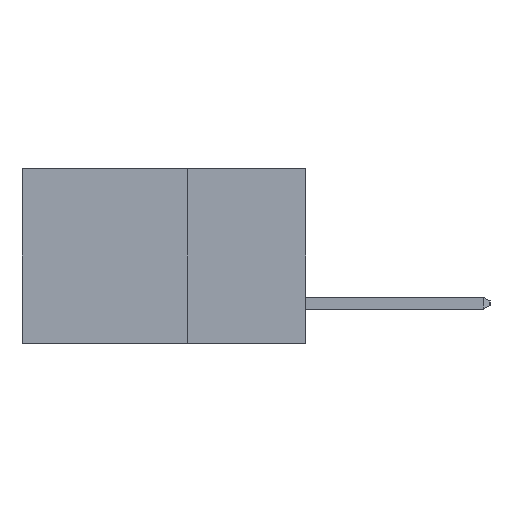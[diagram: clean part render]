
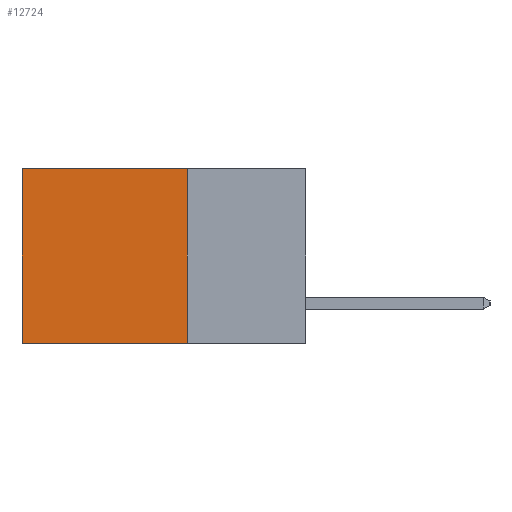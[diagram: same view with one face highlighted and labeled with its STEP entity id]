
A CAD part, left-side view. The second image highlights one B-rep face of the part: STEP entity #12724.
In plain terms, the highlighted planar face has unit normal (-1, 0, 0).
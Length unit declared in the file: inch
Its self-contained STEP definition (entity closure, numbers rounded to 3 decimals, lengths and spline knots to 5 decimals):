
#132 = CARTESIAN_POINT ( 'NONE',  ( 0.298, 0.25, 0. ) ) ;
#136 = ORIENTED_EDGE ( 'NONE', *, *, #9781, .F. ) ;
#365 = ORIENTED_EDGE ( 'NONE', *, *, #11097, .F. ) ;
#1164 = VERTEX_POINT ( 'NONE', #7019 ) ;
#1993 = EDGE_CURVE ( 'NONE', #12149, #13984, #2616, .T. ) ;
#2065 = AXIS2_PLACEMENT_3D ( 'NONE', #5774, #7041, #15264 ) ;
#2164 = EDGE_CURVE ( 'NONE', #5030, #12149, #10288, .T. ) ;
#2616 = LINE ( 'NONE', #6552, #8946 ) ;
#2800 = VECTOR ( 'NONE', #10578, 39.37008 ) ;
#4017 = CARTESIAN_POINT ( 'NONE',  ( 0.298, 0.25, 0. ) ) ;
#4570 = CARTESIAN_POINT ( 'NONE',  ( 0.298, 0.6, 0. ) ) ;
#5030 = VERTEX_POINT ( 'NONE', #132 ) ;
#5410 = LINE ( 'NONE', #13071, #11493 ) ;
#5774 = CARTESIAN_POINT ( 'NONE',  ( 0.298, 0.25, 0. ) ) ;
#6486 = DIRECTION ( 'NONE',  ( 0., 0., -1. ) ) ;
#6552 = CARTESIAN_POINT ( 'NONE',  ( 0.298, 0.6, 0. ) ) ;
#7019 = CARTESIAN_POINT ( 'NONE',  ( 0.298, 0.25, -0.37 ) ) ;
#7041 = DIRECTION ( 'NONE',  ( 1., 0., 0. ) ) ;
#7250 = DIRECTION ( 'NONE',  ( 0., 1., 0. ) ) ;
#7661 = EDGE_LOOP ( 'NONE', ( #11614, #365, #136, #7748 ) ) ;
#7748 = ORIENTED_EDGE ( 'NONE', *, *, #2164, .T. ) ;
#8946 = VECTOR ( 'NONE', #6486, 39.37008 ) ;
#9781 = EDGE_CURVE ( 'NONE', #5030, #1164, #15673, .T. ) ;
#10288 = LINE ( 'NONE', #4017, #12952 ) ;
#10578 = DIRECTION ( 'NONE',  ( 0., 0., -1. ) ) ;
#10664 = CARTESIAN_POINT ( 'NONE',  ( 0.298, 0.25, 0. ) ) ;
#11097 = EDGE_CURVE ( 'NONE', #1164, #13984, #5410, .T. ) ;
#11460 = FACE_OUTER_BOUND ( 'NONE', #7661, .T. ) ;
#11493 = VECTOR ( 'NONE', #12766, 39.37008 ) ;
#11614 = ORIENTED_EDGE ( 'NONE', *, *, #1993, .T. ) ;
#11801 = CARTESIAN_POINT ( 'NONE',  ( 0.298, 0.6, -0.37 ) ) ;
#12149 = VERTEX_POINT ( 'NONE', #4570 ) ;
#12724 = ADVANCED_FACE ( 'NONE', ( #11460 ), #12906, .F. ) ;
#12766 = DIRECTION ( 'NONE',  ( 0., 1., 0. ) ) ;
#12906 = PLANE ( 'NONE',  #2065 ) ;
#12952 = VECTOR ( 'NONE', #7250, 39.37008 ) ;
#13071 = CARTESIAN_POINT ( 'NONE',  ( 0.298, 0.25, -0.37 ) ) ;
#13984 = VERTEX_POINT ( 'NONE', #11801 ) ;
#15264 = DIRECTION ( 'NONE',  ( 0., 0., -1. ) ) ;
#15673 = LINE ( 'NONE', #10664, #2800 ) ;
